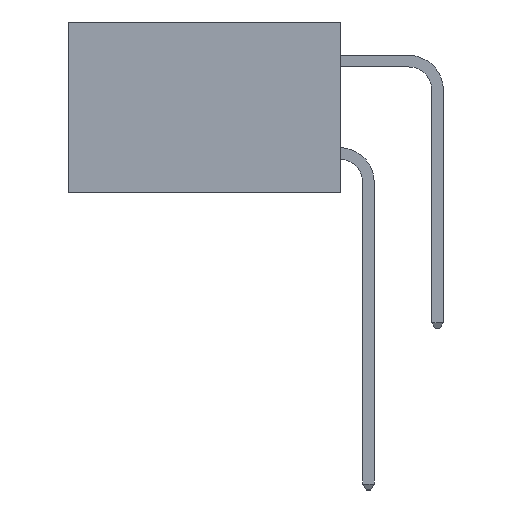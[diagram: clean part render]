
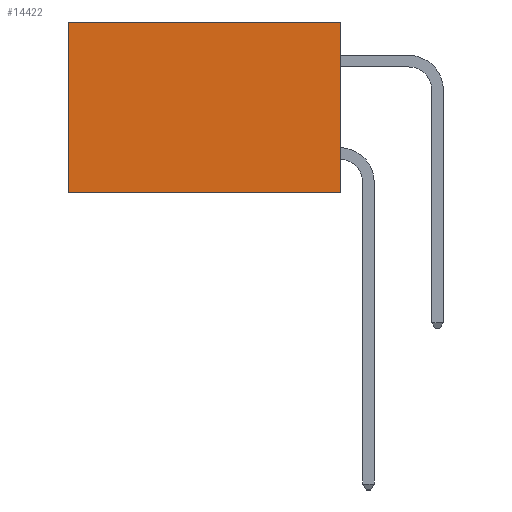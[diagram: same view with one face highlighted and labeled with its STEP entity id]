
A CAD part, left-side view. The second image highlights one B-rep face of the part: STEP entity #14422.
In plain terms, the highlighted planar face has unit normal (-1, 0, 0).
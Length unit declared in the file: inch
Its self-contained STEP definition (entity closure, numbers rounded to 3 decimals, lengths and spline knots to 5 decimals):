
#2115 = LINE ( 'NONE', #26190, #13049 ) ;
#2501 = VERTEX_POINT ( 'NONE', #9025 ) ;
#2931 = DIRECTION ( 'NONE',  ( 0., 0., -1. ) ) ;
#3326 = DIRECTION ( 'NONE',  ( 0., 0., -1. ) ) ;
#4631 = VECTOR ( 'NONE', #9769, 39.37008 ) ;
#5065 = CARTESIAN_POINT ( 'NONE',  ( 0.277, 0., 0. ) ) ;
#8180 = ORIENTED_EDGE ( 'NONE', *, *, #20659, .F. ) ;
#9025 = CARTESIAN_POINT ( 'NONE',  ( 0.277, 0., -0.37 ) ) ;
#9769 = DIRECTION ( 'NONE',  ( 0., 1., 0. ) ) ;
#10849 = DIRECTION ( 'NONE',  ( 0., 1., 0. ) ) ;
#13049 = VECTOR ( 'NONE', #14699, 39.37008 ) ;
#13127 = EDGE_CURVE ( 'NONE', #24386, #2501, #25544, .T. ) ;
#13386 = ORIENTED_EDGE ( 'NONE', *, *, #27860, .T. ) ;
#13713 = EDGE_LOOP ( 'NONE', ( #13386, #8180, #16308, #26389 ) ) ;
#14422 = ADVANCED_FACE ( 'NONE', ( #25880 ), #26016, .F. ) ;
#14471 = VECTOR ( 'NONE', #10849, 39.37008 ) ;
#14699 = DIRECTION ( 'NONE',  ( 0., 0., -1. ) ) ;
#15379 = CARTESIAN_POINT ( 'NONE',  ( 0.277, 0., -0.37 ) ) ;
#16308 = ORIENTED_EDGE ( 'NONE', *, *, #13127, .F. ) ;
#16827 = DIRECTION ( 'NONE',  ( 1., 0., 0. ) ) ;
#17743 = CARTESIAN_POINT ( 'NONE',  ( 0.277, 0.59, 0. ) ) ;
#20659 = EDGE_CURVE ( 'NONE', #2501, #22675, #26755, .T. ) ;
#21594 = CARTESIAN_POINT ( 'NONE',  ( 0.277, 0., 0. ) ) ;
#22102 = EDGE_CURVE ( 'NONE', #24386, #26777, #23033, .T. ) ;
#22675 = VERTEX_POINT ( 'NONE', #26955 ) ;
#23033 = LINE ( 'NONE', #5065, #4631 ) ;
#24386 = VERTEX_POINT ( 'NONE', #21594 ) ;
#24824 = VECTOR ( 'NONE', #3326, 39.37008 ) ;
#25544 = LINE ( 'NONE', #26387, #24824 ) ;
#25880 = FACE_OUTER_BOUND ( 'NONE', #13713, .T. ) ;
#26016 = PLANE ( 'NONE',  #26277 ) ;
#26190 = CARTESIAN_POINT ( 'NONE',  ( 0.277, 0.59, -0.37 ) ) ;
#26277 = AXIS2_PLACEMENT_3D ( 'NONE', #28329, #16827, #2931 ) ;
#26387 = CARTESIAN_POINT ( 'NONE',  ( 0.277, 0., -0.37 ) ) ;
#26389 = ORIENTED_EDGE ( 'NONE', *, *, #22102, .T. ) ;
#26755 = LINE ( 'NONE', #15379, #14471 ) ;
#26777 = VERTEX_POINT ( 'NONE', #17743 ) ;
#26955 = CARTESIAN_POINT ( 'NONE',  ( 0.277, 0.59, -0.37 ) ) ;
#27860 = EDGE_CURVE ( 'NONE', #26777, #22675, #2115, .T. ) ;
#28329 = CARTESIAN_POINT ( 'NONE',  ( 0.277, 0., -0.37 ) ) ;
